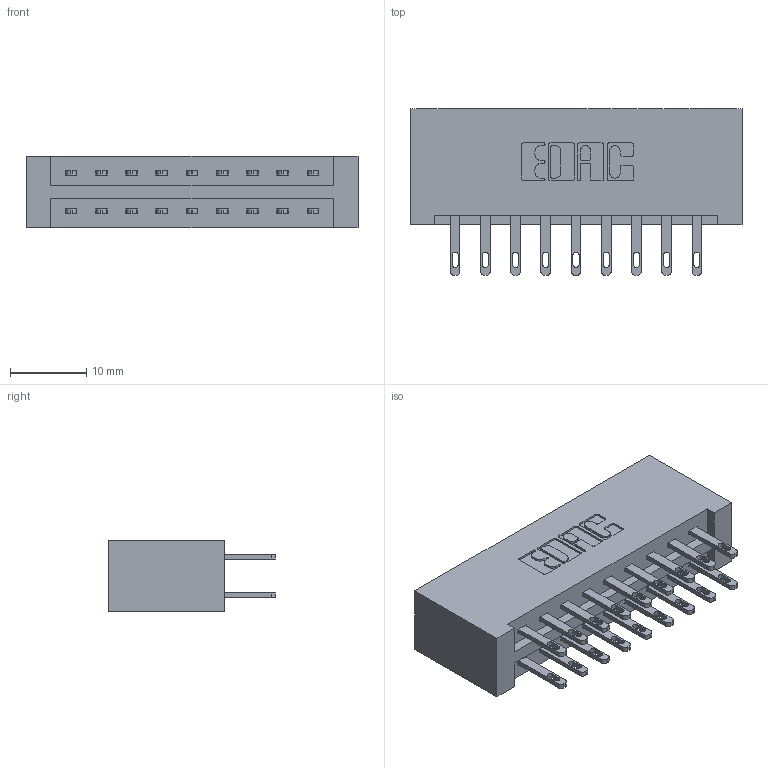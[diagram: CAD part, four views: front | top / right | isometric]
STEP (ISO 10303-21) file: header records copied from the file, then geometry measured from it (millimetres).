
FILE_DESCRIPTION (( 'STEP AP203' ), '1' );
FILE_NAME ('337-018-500-201.STEP', '2019-10-08T12:52:05', ( '' ), ( '' ), 'SwSTEP 2.0', 'SolidWorks 2016', '' );
FILE_SCHEMA (( 'CONFIG_CONTROL_DESIGN' ));
Length unit declared in the file: inch
Products named in the file (3): 345-292-001_345-293-100; 337-018-500-201; 337 Part_No Mounting Lugs
Assembly tree (19 placements, depth 2):
  337-018-500-201
    337 Part_No Mounting Lugs
    345-292-001_345-293-100  x18
Bounding box: 43.54 x 21.85 x 9.4 mm (x, y, z)
Volume: 4964.6 mm3; surface area: 5547.8 mm2
Topology: 19 solids, 19 shells, 1006 faces, 3041 edges, 2026 vertices
Faces by surface type: plane 642, cylinder 364
Entity records: 10899 total; most frequent: CARTESIAN_POINT 1862, ORIENTED_EDGE 1798, DIRECTION 1639, EDGE_CURVE 899, VECTOR 775, LINE 775, VERTEX_POINT 598, AXIS2_PLACEMENT_3D 432
